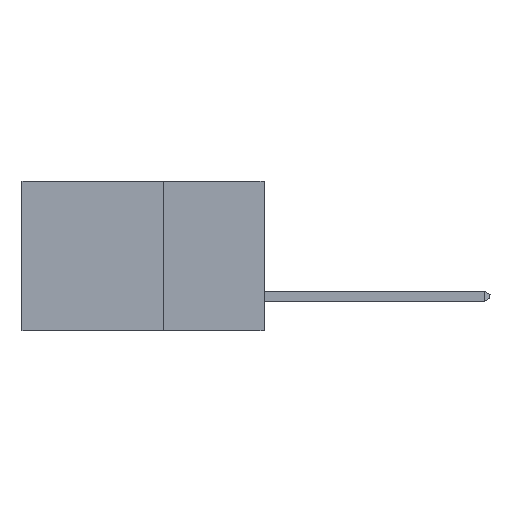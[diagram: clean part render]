
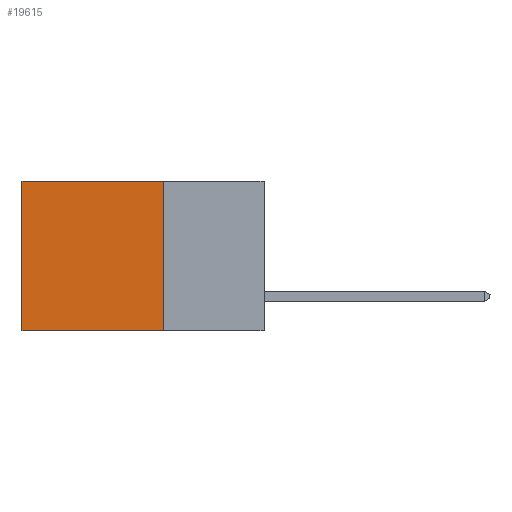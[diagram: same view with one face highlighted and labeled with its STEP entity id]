
A CAD part, left-side view. The second image highlights one B-rep face of the part: STEP entity #19615.
In plain terms, the highlighted planar face has unit normal (-1, 0, 0).
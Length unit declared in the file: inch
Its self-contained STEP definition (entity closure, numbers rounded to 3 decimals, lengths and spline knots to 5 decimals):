
#1198 = EDGE_CURVE ( 'NONE', #18536, #17425, #7977, .T. ) ;
#2143 = DIRECTION ( 'NONE',  ( 0., 1., 0. ) ) ;
#2227 = VECTOR ( 'NONE', #9610, 39.37008 ) ;
#2995 = DIRECTION ( 'NONE',  ( 0., 0., -1. ) ) ;
#3062 = DIRECTION ( 'NONE',  ( 0., 0., -1. ) ) ;
#3583 = CARTESIAN_POINT ( 'NONE',  ( 0.2615, 0.25, -0.37 ) ) ;
#3685 = VECTOR ( 'NONE', #2995, 39.37008 ) ;
#3914 = LINE ( 'NONE', #14096, #14768 ) ;
#4094 = ORIENTED_EDGE ( 'NONE', *, *, #18453, .T. ) ;
#4554 = PLANE ( 'NONE',  #19674 ) ;
#6437 = DIRECTION ( 'NONE',  ( 0., 0., -1. ) ) ;
#7094 = EDGE_LOOP ( 'NONE', ( #20745, #12221, #20338, #4094 ) ) ;
#7764 = CARTESIAN_POINT ( 'NONE',  ( 0.2615, 0.6, -0.37 ) ) ;
#7942 = CARTESIAN_POINT ( 'NONE',  ( 0.2615, 0.25, -0.37 ) ) ;
#7977 = LINE ( 'NONE', #16499, #3685 ) ;
#8038 = CARTESIAN_POINT ( 'NONE',  ( 0.2615, 0.25, 0. ) ) ;
#9114 = VECTOR ( 'NONE', #3062, 39.37008 ) ;
#9610 = DIRECTION ( 'NONE',  ( 0., 1., 0. ) ) ;
#9864 = DIRECTION ( 'NONE',  ( 1., 0., 0. ) ) ;
#9878 = VERTEX_POINT ( 'NONE', #3583 ) ;
#9911 = EDGE_CURVE ( 'NONE', #17167, #9878, #16360, .T. ) ;
#10050 = EDGE_CURVE ( 'NONE', #9878, #17425, #3914, .T. ) ;
#12221 = ORIENTED_EDGE ( 'NONE', *, *, #10050, .F. ) ;
#13059 = CARTESIAN_POINT ( 'NONE',  ( 0.2615, 0.25, -0.37 ) ) ;
#14096 = CARTESIAN_POINT ( 'NONE',  ( 0.2615, 0.25, -0.37 ) ) ;
#14719 = FACE_OUTER_BOUND ( 'NONE', #7094, .T. ) ;
#14768 = VECTOR ( 'NONE', #2143, 39.37008 ) ;
#16009 = CARTESIAN_POINT ( 'NONE',  ( 0.2615, 0.6, 0. ) ) ;
#16360 = LINE ( 'NONE', #7942, #9114 ) ;
#16499 = CARTESIAN_POINT ( 'NONE',  ( 0.2615, 0.6, -0.37 ) ) ;
#17167 = VERTEX_POINT ( 'NONE', #21376 ) ;
#17425 = VERTEX_POINT ( 'NONE', #7764 ) ;
#18453 = EDGE_CURVE ( 'NONE', #17167, #18536, #19646, .T. ) ;
#18536 = VERTEX_POINT ( 'NONE', #16009 ) ;
#19615 = ADVANCED_FACE ( 'NONE', ( #14719 ), #4554, .F. ) ;
#19646 = LINE ( 'NONE', #8038, #2227 ) ;
#19674 = AXIS2_PLACEMENT_3D ( 'NONE', #13059, #9864, #6437 ) ;
#20338 = ORIENTED_EDGE ( 'NONE', *, *, #9911, .F. ) ;
#20745 = ORIENTED_EDGE ( 'NONE', *, *, #1198, .T. ) ;
#21376 = CARTESIAN_POINT ( 'NONE',  ( 0.2615, 0.25, 0. ) ) ;
